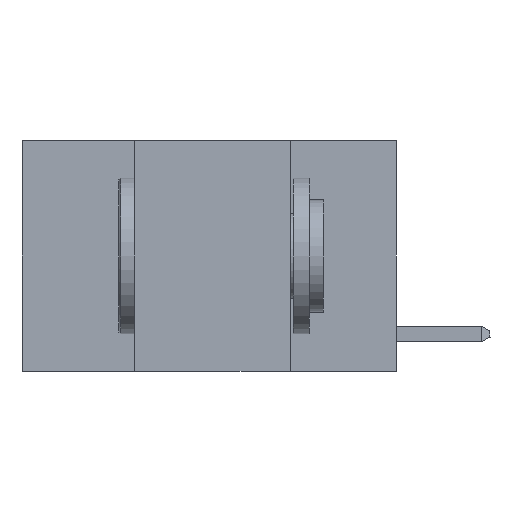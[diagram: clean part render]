
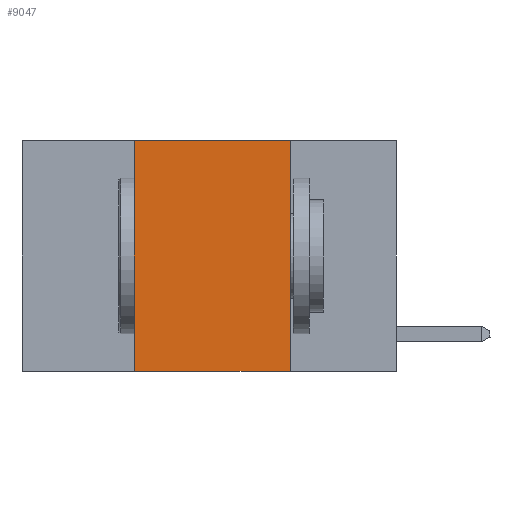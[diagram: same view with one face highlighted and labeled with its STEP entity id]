
A CAD part, left-side view. The second image highlights one B-rep face of the part: STEP entity #9047.
In plain terms, the highlighted planar face has unit normal (-1, 0, 0).
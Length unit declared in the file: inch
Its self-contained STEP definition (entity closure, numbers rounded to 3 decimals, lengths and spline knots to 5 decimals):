
#234 = LINE ( 'NONE', #1785, #2141 ) ;
#267 = DIRECTION ( 'NONE',  ( 0., 0., -1. ) ) ;
#601 = VERTEX_POINT ( 'NONE', #1259 ) ;
#1202 = VECTOR ( 'NONE', #1945, 39.37008 ) ;
#1259 = CARTESIAN_POINT ( 'NONE',  ( 0., 0.17, -0.37 ) ) ;
#1785 = CARTESIAN_POINT ( 'NONE',  ( 0., 0.6, -0.37 ) ) ;
#1793 = CARTESIAN_POINT ( 'NONE',  ( 0., 0.42, 0. ) ) ;
#1849 = VECTOR ( 'NONE', #267, 39.37008 ) ;
#1918 = CARTESIAN_POINT ( 'NONE',  ( 0., 0.6, 0. ) ) ;
#1945 = DIRECTION ( 'NONE',  ( 0., -1., 0. ) ) ;
#1961 = VECTOR ( 'NONE', #4268, 39.37008 ) ;
#2110 = EDGE_CURVE ( 'NONE', #7251, #601, #7921, .T. ) ;
#2141 = VECTOR ( 'NONE', #6396, 39.37008 ) ;
#2224 = EDGE_LOOP ( 'NONE', ( #5169, #5563, #2416, #9723 ) ) ;
#2322 = VERTEX_POINT ( 'NONE', #3906 ) ;
#2416 = ORIENTED_EDGE ( 'NONE', *, *, #2527, .F. ) ;
#2527 = EDGE_CURVE ( 'NONE', #2322, #8841, #6079, .T. ) ;
#2821 = CARTESIAN_POINT ( 'NONE',  ( 0., 0.6, 0. ) ) ;
#3195 = EDGE_CURVE ( 'NONE', #8841, #7251, #9286, .T. ) ;
#3906 = CARTESIAN_POINT ( 'NONE',  ( 0., 0.42, -0.37 ) ) ;
#4268 = DIRECTION ( 'NONE',  ( 0., 0., 1. ) ) ;
#5169 = ORIENTED_EDGE ( 'NONE', *, *, #2110, .F. ) ;
#5195 = DIRECTION ( 'NONE',  ( 0., 0., -1. ) ) ;
#5561 = FACE_OUTER_BOUND ( 'NONE', #2224, .T. ) ;
#5563 = ORIENTED_EDGE ( 'NONE', *, *, #3195, .F. ) ;
#6079 = LINE ( 'NONE', #6464, #1961 ) ;
#6396 = DIRECTION ( 'NONE',  ( 0., -1., 0. ) ) ;
#6464 = CARTESIAN_POINT ( 'NONE',  ( 0., 0.42, 0. ) ) ;
#6471 = CARTESIAN_POINT ( 'NONE',  ( 0., 0.17, 0. ) ) ;
#7251 = VERTEX_POINT ( 'NONE', #9678 ) ;
#7573 = EDGE_CURVE ( 'NONE', #2322, #601, #234, .T. ) ;
#7921 = LINE ( 'NONE', #6471, #1849 ) ;
#8340 = AXIS2_PLACEMENT_3D ( 'NONE', #2821, #9573, #5195 ) ;
#8841 = VERTEX_POINT ( 'NONE', #1793 ) ;
#8846 = PLANE ( 'NONE',  #8340 ) ;
#9047 = ADVANCED_FACE ( 'NONE', ( #5561 ), #8846, .F. ) ;
#9286 = LINE ( 'NONE', #1918, #1202 ) ;
#9573 = DIRECTION ( 'NONE',  ( 1., 0., 0. ) ) ;
#9678 = CARTESIAN_POINT ( 'NONE',  ( 0., 0.17, 0. ) ) ;
#9723 = ORIENTED_EDGE ( 'NONE', *, *, #7573, .T. ) ;
